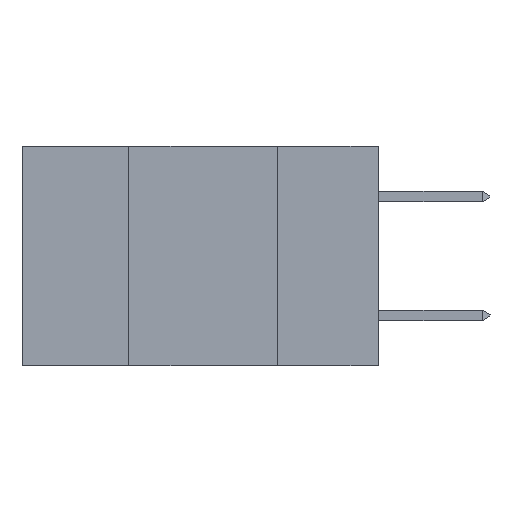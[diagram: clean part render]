
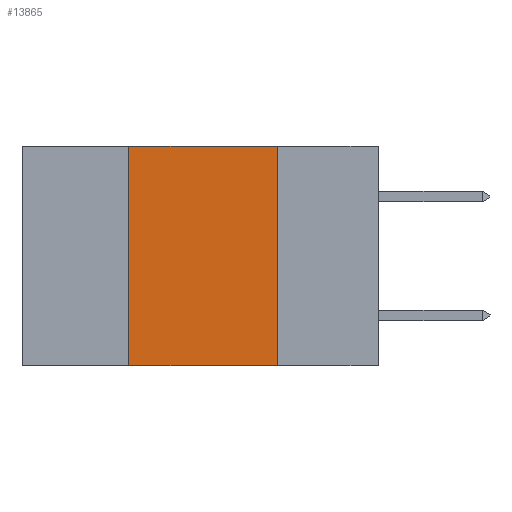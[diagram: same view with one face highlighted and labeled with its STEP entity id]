
A CAD part, left-side view. The second image highlights one B-rep face of the part: STEP entity #13865.
In plain terms, the highlighted planar face has unit normal (-1, 0, 0).
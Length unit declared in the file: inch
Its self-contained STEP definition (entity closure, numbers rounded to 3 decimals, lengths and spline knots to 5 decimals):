
#86 = VERTEX_POINT ( 'NONE', #16258 ) ;
#422 = VECTOR ( 'NONE', #7660, 39.37008 ) ;
#1265 = DIRECTION ( 'NONE',  ( 0., 0., 1. ) ) ;
#1307 = EDGE_CURVE ( 'NONE', #2920, #4636, #11756, .T. ) ;
#1316 = VECTOR ( 'NONE', #6740, 39.37008 ) ;
#1574 = VECTOR ( 'NONE', #6968, 39.37008 ) ;
#2058 = EDGE_CURVE ( 'NONE', #2920, #9240, #8443, .T. ) ;
#2920 = VERTEX_POINT ( 'NONE', #9981 ) ;
#3347 = EDGE_CURVE ( 'NONE', #86, #9240, #9020, .T. ) ;
#4636 = VERTEX_POINT ( 'NONE', #12056 ) ;
#5874 = PLANE ( 'NONE',  #9324 ) ;
#6269 = EDGE_LOOP ( 'NONE', ( #12450, #16896, #13438, #11474 ) ) ;
#6740 = DIRECTION ( 'NONE',  ( 0., 0., -1. ) ) ;
#6801 = CARTESIAN_POINT ( 'NONE',  ( 0., 0.17, -0.37 ) ) ;
#6968 = DIRECTION ( 'NONE',  ( 0., -1., 0. ) ) ;
#7336 = LINE ( 'NONE', #10342, #422 ) ;
#7660 = DIRECTION ( 'NONE',  ( 0., -1., 0. ) ) ;
#7710 = EDGE_CURVE ( 'NONE', #4636, #86, #7336, .T. ) ;
#7772 = CARTESIAN_POINT ( 'NONE',  ( 0., 0.42, 0. ) ) ;
#8443 = LINE ( 'NONE', #11100, #1574 ) ;
#9020 = LINE ( 'NONE', #15946, #1316 ) ;
#9240 = VERTEX_POINT ( 'NONE', #6801 ) ;
#9324 = AXIS2_PLACEMENT_3D ( 'NONE', #12624, #15159, #15318 ) ;
#9981 = CARTESIAN_POINT ( 'NONE',  ( 0., 0.42, -0.37 ) ) ;
#10342 = CARTESIAN_POINT ( 'NONE',  ( 0., 0.6, 0. ) ) ;
#11100 = CARTESIAN_POINT ( 'NONE',  ( 0., 0.6, -0.37 ) ) ;
#11474 = ORIENTED_EDGE ( 'NONE', *, *, #2058, .T. ) ;
#11756 = LINE ( 'NONE', #7772, #16075 ) ;
#12056 = CARTESIAN_POINT ( 'NONE',  ( 0., 0.42, 0. ) ) ;
#12450 = ORIENTED_EDGE ( 'NONE', *, *, #3347, .F. ) ;
#12624 = CARTESIAN_POINT ( 'NONE',  ( 0., 0.6, 0. ) ) ;
#13438 = ORIENTED_EDGE ( 'NONE', *, *, #1307, .F. ) ;
#13865 = ADVANCED_FACE ( 'NONE', ( #16232 ), #5874, .F. ) ;
#15159 = DIRECTION ( 'NONE',  ( 1., 0., 0. ) ) ;
#15318 = DIRECTION ( 'NONE',  ( 0., 0., -1. ) ) ;
#15946 = CARTESIAN_POINT ( 'NONE',  ( 0., 0.17, 0. ) ) ;
#16075 = VECTOR ( 'NONE', #1265, 39.37008 ) ;
#16232 = FACE_OUTER_BOUND ( 'NONE', #6269, .T. ) ;
#16258 = CARTESIAN_POINT ( 'NONE',  ( 0., 0.17, 0. ) ) ;
#16896 = ORIENTED_EDGE ( 'NONE', *, *, #7710, .F. ) ;
